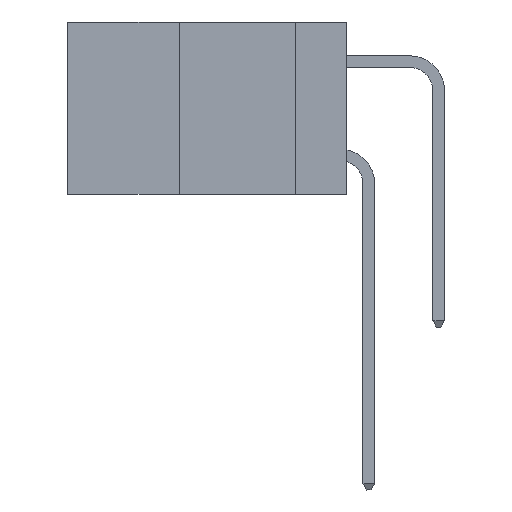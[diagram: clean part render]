
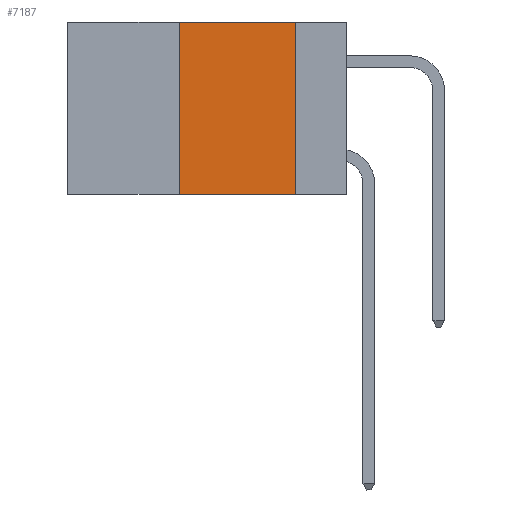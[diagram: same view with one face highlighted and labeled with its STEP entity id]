
A CAD part, left-side view. The second image highlights one B-rep face of the part: STEP entity #7187.
In plain terms, the highlighted planar face has unit normal (-1, 0, 0).
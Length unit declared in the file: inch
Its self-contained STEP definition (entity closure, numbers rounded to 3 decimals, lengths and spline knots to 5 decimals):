
#747 = VECTOR ( 'NONE', #4183, 39.37008 ) ;
#842 = VERTEX_POINT ( 'NONE', #5039 ) ;
#936 = DIRECTION ( 'NONE',  ( 0., 0., -1. ) ) ;
#1134 = VERTEX_POINT ( 'NONE', #7949 ) ;
#1580 = DIRECTION ( 'NONE',  ( 0., 0., 1. ) ) ;
#2543 = VERTEX_POINT ( 'NONE', #12446 ) ;
#2756 = ORIENTED_EDGE ( 'NONE', *, *, #8983, .T. ) ;
#3109 = CARTESIAN_POINT ( 'NONE',  ( 0., 0.6, 0. ) ) ;
#3112 = CARTESIAN_POINT ( 'NONE',  ( 0., 0.6, -0.37 ) ) ;
#3491 = DIRECTION ( 'NONE',  ( 0., 0., -1. ) ) ;
#3543 = VERTEX_POINT ( 'NONE', #5140 ) ;
#3556 = VECTOR ( 'NONE', #1580, 39.37008 ) ;
#4183 = DIRECTION ( 'NONE',  ( 0., -1., 0. ) ) ;
#4242 = AXIS2_PLACEMENT_3D ( 'NONE', #3109, #7288, #936 ) ;
#5039 = CARTESIAN_POINT ( 'NONE',  ( 0., 0.36, -0.37 ) ) ;
#5110 = ORIENTED_EDGE ( 'NONE', *, *, #5997, .F. ) ;
#5140 = CARTESIAN_POINT ( 'NONE',  ( 0., 0.11, -0.37 ) ) ;
#5696 = VECTOR ( 'NONE', #3491, 39.37008 ) ;
#5729 = EDGE_CURVE ( 'NONE', #1134, #2543, #12869, .T. ) ;
#5997 = EDGE_CURVE ( 'NONE', #2543, #3543, #10117, .T. ) ;
#6126 = CARTESIAN_POINT ( 'NONE',  ( 0., 0.6, 0. ) ) ;
#6302 = LINE ( 'NONE', #11821, #3556 ) ;
#7187 = ADVANCED_FACE ( 'NONE', ( #12535 ), #11266, .F. ) ;
#7288 = DIRECTION ( 'NONE',  ( 1., 0., 0. ) ) ;
#7633 = VECTOR ( 'NONE', #8227, 39.37008 ) ;
#7949 = CARTESIAN_POINT ( 'NONE',  ( 0., 0.36, 0. ) ) ;
#8227 = DIRECTION ( 'NONE',  ( 0., -1., 0. ) ) ;
#8983 = EDGE_CURVE ( 'NONE', #842, #3543, #11760, .T. ) ;
#9315 = ORIENTED_EDGE ( 'NONE', *, *, #5729, .F. ) ;
#10117 = LINE ( 'NONE', #10602, #5696 ) ;
#10602 = CARTESIAN_POINT ( 'NONE',  ( 0., 0.11, 0. ) ) ;
#10814 = ORIENTED_EDGE ( 'NONE', *, *, #12267, .F. ) ;
#11266 = PLANE ( 'NONE',  #4242 ) ;
#11760 = LINE ( 'NONE', #3112, #747 ) ;
#11821 = CARTESIAN_POINT ( 'NONE',  ( 0., 0.36, 0. ) ) ;
#12076 = EDGE_LOOP ( 'NONE', ( #5110, #9315, #10814, #2756 ) ) ;
#12267 = EDGE_CURVE ( 'NONE', #842, #1134, #6302, .T. ) ;
#12446 = CARTESIAN_POINT ( 'NONE',  ( 0., 0.11, 0. ) ) ;
#12535 = FACE_OUTER_BOUND ( 'NONE', #12076, .T. ) ;
#12869 = LINE ( 'NONE', #6126, #7633 ) ;
